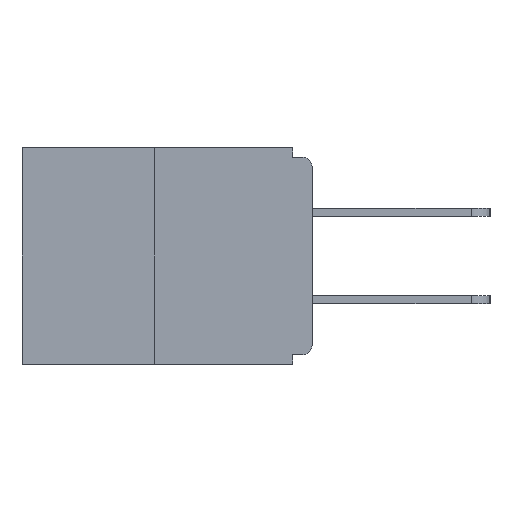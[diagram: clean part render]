
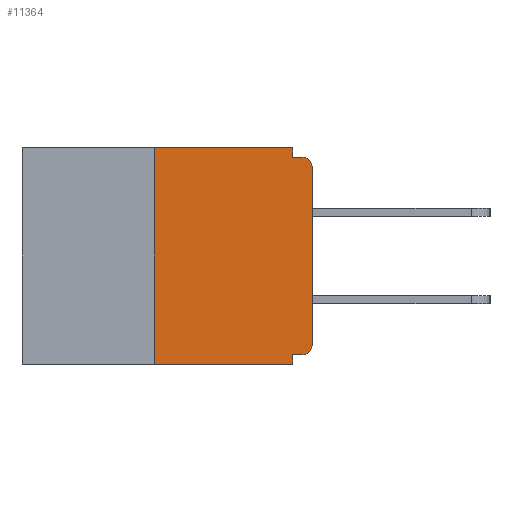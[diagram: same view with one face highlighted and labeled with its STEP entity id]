
A CAD part, left-side view. The second image highlights one B-rep face of the part: STEP entity #11364.
In plain terms, the highlighted planar face has unit normal (-1, 0, 0).
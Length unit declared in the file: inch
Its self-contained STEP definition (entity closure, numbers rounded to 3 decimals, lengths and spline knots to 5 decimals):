
#312 = EDGE_CURVE ( 'NONE', #8785, #6707, #8220, .T. ) ;
#643 = CARTESIAN_POINT ( 'NONE',  ( 0., 0.015, -0.313 ) ) ;
#675 = ORIENTED_EDGE ( 'NONE', *, *, #9790, .T. ) ;
#727 = VECTOR ( 'NONE', #6609, 39.37008 ) ;
#1130 = ORIENTED_EDGE ( 'NONE', *, *, #1161, .T. ) ;
#1161 = EDGE_CURVE ( 'NONE', #3624, #6707, #8577, .T. ) ;
#1322 = ORIENTED_EDGE ( 'NONE', *, *, #6853, .F. ) ;
#1428 = DIRECTION ( 'NONE',  ( 0., 0., -1. ) ) ;
#1545 = CARTESIAN_POINT ( 'NONE',  ( 0., 0.015, -0.328 ) ) ;
#1568 = DIRECTION ( 'NONE',  ( 0., -1., 0. ) ) ;
#1578 = CARTESIAN_POINT ( 'NONE',  ( 0., 0., 0. ) ) ;
#1739 = EDGE_CURVE ( 'NONE', #14441, #14473, #6532, .T. ) ;
#1757 = DIRECTION ( 'NONE',  ( 0., 0., -1. ) ) ;
#2285 = VECTOR ( 'NONE', #5107, 39.37008 ) ;
#2375 = LINE ( 'NONE', #13723, #5091 ) ;
#2545 = CARTESIAN_POINT ( 'NONE',  ( 0., 0.015, -0.015 ) ) ;
#2920 = VERTEX_POINT ( 'NONE', #1545 ) ;
#3174 = VECTOR ( 'NONE', #1568, 39.37008 ) ;
#3624 = VERTEX_POINT ( 'NONE', #10623 ) ;
#3641 = VERTEX_POINT ( 'NONE', #12036 ) ;
#3840 = CARTESIAN_POINT ( 'NONE',  ( 0., 0.031, -0.015 ) ) ;
#4016 = ORIENTED_EDGE ( 'NONE', *, *, #13500, .T. ) ;
#4288 = CARTESIAN_POINT ( 'NONE',  ( 0., 0.25, 0. ) ) ;
#4448 = LINE ( 'NONE', #1578, #2285 ) ;
#4889 = AXIS2_PLACEMENT_3D ( 'NONE', #643, #5245, #1757 ) ;
#4926 = CARTESIAN_POINT ( 'NONE',  ( 0., 0.46, 0. ) ) ;
#4966 = CARTESIAN_POINT ( 'NONE',  ( 0., 0.015, -0.03 ) ) ;
#5091 = VECTOR ( 'NONE', #12619, 39.37008 ) ;
#5107 = DIRECTION ( 'NONE',  ( 0., 0., 1. ) ) ;
#5245 = DIRECTION ( 'NONE',  ( -1., 0., 0. ) ) ;
#5261 = EDGE_CURVE ( 'NONE', #12439, #12693, #6792, .T. ) ;
#5347 = CARTESIAN_POINT ( 'NONE',  ( 0., 0.031, -0.343 ) ) ;
#5922 = AXIS2_PLACEMENT_3D ( 'NONE', #4966, #6087, #1428 ) ;
#6087 = DIRECTION ( 'NONE',  ( -1., 0., 0. ) ) ;
#6137 = DIRECTION ( 'NONE',  ( 1., 0., 0. ) ) ;
#6280 = CARTESIAN_POINT ( 'NONE',  ( 0., 0.46, -0.343 ) ) ;
#6282 = LINE ( 'NONE', #6280, #3174 ) ;
#6532 = LINE ( 'NONE', #5347, #11088 ) ;
#6609 = DIRECTION ( 'NONE',  ( 0., 0., 1. ) ) ;
#6707 = VERTEX_POINT ( 'NONE', #2545 ) ;
#6757 = CARTESIAN_POINT ( 'NONE',  ( 0., 0., -0.015 ) ) ;
#6792 = LINE ( 'NONE', #4926, #13321 ) ;
#6853 = EDGE_CURVE ( 'NONE', #12693, #8785, #2375, .T. ) ;
#7085 = DIRECTION ( 'NONE',  ( 0., 1., 0. ) ) ;
#7263 = FACE_OUTER_BOUND ( 'NONE', #9958, .T. ) ;
#7437 = CIRCLE ( 'NONE', #4889, 0.015 ) ;
#7490 = VECTOR ( 'NONE', #11433, 39.37008 ) ;
#7878 = CARTESIAN_POINT ( 'NONE',  ( 0., 0.25, 0. ) ) ;
#8220 = LINE ( 'NONE', #6757, #7490 ) ;
#8374 = VERTEX_POINT ( 'NONE', #8508 ) ;
#8508 = CARTESIAN_POINT ( 'NONE',  ( 0., 0., -0.313 ) ) ;
#8536 = EDGE_CURVE ( 'NONE', #2920, #8374, #7437, .T. ) ;
#8577 = CIRCLE ( 'NONE', #5922, 0.015 ) ;
#8579 = AXIS2_PLACEMENT_3D ( 'NONE', #8630, #6137, #10885 ) ;
#8630 = CARTESIAN_POINT ( 'NONE',  ( 0., 0.46, 0. ) ) ;
#8785 = VERTEX_POINT ( 'NONE', #3840 ) ;
#9455 = LINE ( 'NONE', #4288, #727 ) ;
#9662 = CARTESIAN_POINT ( 'NONE',  ( 0., 0.031, -0.343 ) ) ;
#9704 = ORIENTED_EDGE ( 'NONE', *, *, #5261, .F. ) ;
#9790 = EDGE_CURVE ( 'NONE', #8374, #3624, #4448, .T. ) ;
#9958 = EDGE_LOOP ( 'NONE', ( #9704, #13302, #4016, #11901, #13796, #10700, #675, #1130, #14478, #1322 ) ) ;
#10047 = EDGE_CURVE ( 'NONE', #2920, #14441, #13695, .T. ) ;
#10623 = CARTESIAN_POINT ( 'NONE',  ( 0., 0., -0.03 ) ) ;
#10700 = ORIENTED_EDGE ( 'NONE', *, *, #8536, .T. ) ;
#10885 = DIRECTION ( 'NONE',  ( 0., 0., -1. ) ) ;
#11088 = VECTOR ( 'NONE', #14472, 39.37008 ) ;
#11364 = ADVANCED_FACE ( 'NONE', ( #7263 ), #13145, .F. ) ;
#11433 = DIRECTION ( 'NONE',  ( 0., -1., 0. ) ) ;
#11788 = EDGE_CURVE ( 'NONE', #3641, #12439, #9455, .T. ) ;
#11901 = ORIENTED_EDGE ( 'NONE', *, *, #1739, .F. ) ;
#11909 = CARTESIAN_POINT ( 'NONE',  ( 0., 0., -0.328 ) ) ;
#12036 = CARTESIAN_POINT ( 'NONE',  ( 0., 0.25, -0.343 ) ) ;
#12130 = VECTOR ( 'NONE', #7085, 39.37008 ) ;
#12439 = VERTEX_POINT ( 'NONE', #7878 ) ;
#12619 = DIRECTION ( 'NONE',  ( 0., 0., -1. ) ) ;
#12693 = VERTEX_POINT ( 'NONE', #14238 ) ;
#13059 = DIRECTION ( 'NONE',  ( 0., -1., 0. ) ) ;
#13145 = PLANE ( 'NONE',  #8579 ) ;
#13302 = ORIENTED_EDGE ( 'NONE', *, *, #11788, .F. ) ;
#13321 = VECTOR ( 'NONE', #13059, 39.37008 ) ;
#13500 = EDGE_CURVE ( 'NONE', #3641, #14473, #6282, .T. ) ;
#13695 = LINE ( 'NONE', #11909, #12130 ) ;
#13723 = CARTESIAN_POINT ( 'NONE',  ( 0., 0.031, 0. ) ) ;
#13796 = ORIENTED_EDGE ( 'NONE', *, *, #10047, .F. ) ;
#14238 = CARTESIAN_POINT ( 'NONE',  ( 0., 0.031, 0. ) ) ;
#14441 = VERTEX_POINT ( 'NONE', #14909 ) ;
#14472 = DIRECTION ( 'NONE',  ( 0., 0., -1. ) ) ;
#14473 = VERTEX_POINT ( 'NONE', #9662 ) ;
#14478 = ORIENTED_EDGE ( 'NONE', *, *, #312, .F. ) ;
#14909 = CARTESIAN_POINT ( 'NONE',  ( 0., 0.031, -0.328 ) ) ;
